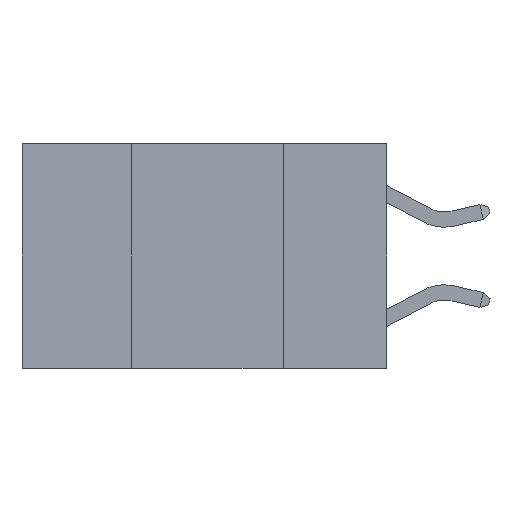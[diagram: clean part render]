
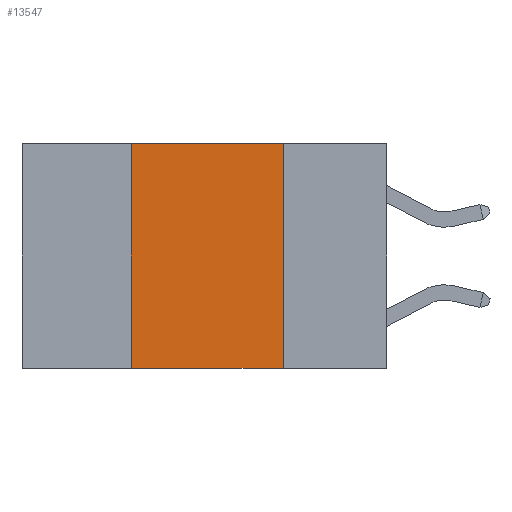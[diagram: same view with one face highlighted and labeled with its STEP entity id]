
A CAD part, left-side view. The second image highlights one B-rep face of the part: STEP entity #13547.
In plain terms, the highlighted planar face has unit normal (-1, 0, 0).
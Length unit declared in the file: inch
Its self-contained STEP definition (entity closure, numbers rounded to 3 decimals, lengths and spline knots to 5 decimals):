
#304 = VERTEX_POINT ( 'NONE', #10022 ) ;
#1421 = DIRECTION ( 'NONE',  ( 0., 0., -1. ) ) ;
#1948 = CARTESIAN_POINT ( 'NONE',  ( 0., 0.42, 0. ) ) ;
#2151 = DIRECTION ( 'NONE',  ( 0., -1., 0. ) ) ;
#2727 = EDGE_CURVE ( 'NONE', #5891, #4727, #16932, .T. ) ;
#4139 = CARTESIAN_POINT ( 'NONE',  ( 0., 0.6, 0. ) ) ;
#4727 = VERTEX_POINT ( 'NONE', #19688 ) ;
#5351 = EDGE_CURVE ( 'NONE', #5891, #304, #20452, .T. ) ;
#5479 = ORIENTED_EDGE ( 'NONE', *, *, #2727, .F. ) ;
#5625 = EDGE_CURVE ( 'NONE', #9270, #304, #17870, .T. ) ;
#5891 = VERTEX_POINT ( 'NONE', #27581 ) ;
#8901 = DIRECTION ( 'NONE',  ( 0., 0., -1. ) ) ;
#9270 = VERTEX_POINT ( 'NONE', #24262 ) ;
#10022 = CARTESIAN_POINT ( 'NONE',  ( 0., 0.17, -0.37 ) ) ;
#10675 = DIRECTION ( 'NONE',  ( 0., 0., 1. ) ) ;
#10882 = VECTOR ( 'NONE', #10675, 39.37008 ) ;
#11916 = DIRECTION ( 'NONE',  ( 0., -1., 0. ) ) ;
#12057 = CARTESIAN_POINT ( 'NONE',  ( 0., 0.6, -0.37 ) ) ;
#12858 = FACE_OUTER_BOUND ( 'NONE', #21560, .T. ) ;
#13547 = ADVANCED_FACE ( 'NONE', ( #12858 ), #20969, .F. ) ;
#14535 = VECTOR ( 'NONE', #11916, 39.37008 ) ;
#15023 = CARTESIAN_POINT ( 'NONE',  ( 0., 0.6, 0. ) ) ;
#15185 = CARTESIAN_POINT ( 'NONE',  ( 0., 0.17, 0. ) ) ;
#16932 = LINE ( 'NONE', #1948, #10882 ) ;
#17429 = LINE ( 'NONE', #15023, #25748 ) ;
#17693 = ORIENTED_EDGE ( 'NONE', *, *, #24374, .F. ) ;
#17870 = LINE ( 'NONE', #15185, #24618 ) ;
#18209 = ORIENTED_EDGE ( 'NONE', *, *, #5625, .F. ) ;
#19688 = CARTESIAN_POINT ( 'NONE',  ( 0., 0.42, 0. ) ) ;
#20452 = LINE ( 'NONE', #12057, #14535 ) ;
#20969 = PLANE ( 'NONE',  #25778 ) ;
#21393 = ORIENTED_EDGE ( 'NONE', *, *, #5351, .T. ) ;
#21560 = EDGE_LOOP ( 'NONE', ( #18209, #17693, #5479, #21393 ) ) ;
#24262 = CARTESIAN_POINT ( 'NONE',  ( 0., 0.17, 0. ) ) ;
#24374 = EDGE_CURVE ( 'NONE', #4727, #9270, #17429, .T. ) ;
#24618 = VECTOR ( 'NONE', #8901, 39.37008 ) ;
#25748 = VECTOR ( 'NONE', #2151, 39.37008 ) ;
#25778 = AXIS2_PLACEMENT_3D ( 'NONE', #4139, #27993, #1421 ) ;
#27581 = CARTESIAN_POINT ( 'NONE',  ( 0., 0.42, -0.37 ) ) ;
#27993 = DIRECTION ( 'NONE',  ( 1., 0., 0. ) ) ;
